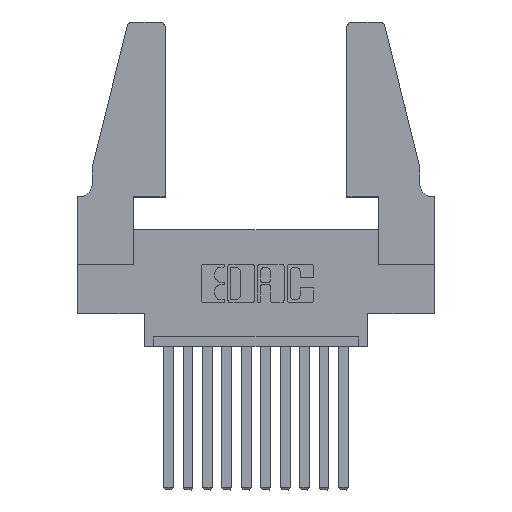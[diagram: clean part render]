
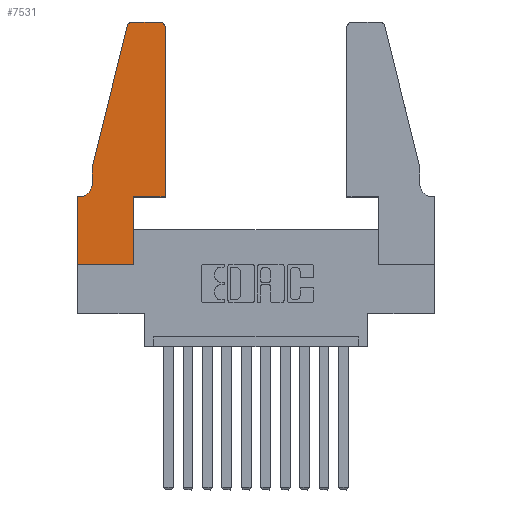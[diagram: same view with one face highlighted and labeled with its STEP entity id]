
A CAD part, top view. The second image highlights one B-rep face of the part: STEP entity #7531.
In plain terms, the highlighted planar face has unit normal (0, 0, 1).
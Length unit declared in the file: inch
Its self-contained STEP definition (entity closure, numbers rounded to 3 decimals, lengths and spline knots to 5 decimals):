
#400 = VERTEX_POINT ( 'NONE', #12386 ) ;
#505 = EDGE_CURVE ( 'NONE', #400, #11823, #3196, .T. ) ;
#638 = VERTEX_POINT ( 'NONE', #8035 ) ;
#693 = EDGE_CURVE ( 'NONE', #10097, #2169, #10620, .T. ) ;
#956 = DIRECTION ( 'NONE',  ( -1., 0., 0. ) ) ;
#965 = VERTEX_POINT ( 'NONE', #2497 ) ;
#1113 = CARTESIAN_POINT ( 'NONE',  ( 0.2605, 1.25, 0.37 ) ) ;
#1134 = CARTESIAN_POINT ( 'NONE',  ( 0.0755, 0.5, 0.37 ) ) ;
#1214 = CARTESIAN_POINT ( 'NONE',  ( 0.4205, 1.22, 0.37 ) ) ;
#1324 = LINE ( 'NONE', #4341, #2148 ) ;
#1554 = ORIENTED_EDGE ( 'NONE', *, *, #2371, .T. ) ;
#1599 = ORIENTED_EDGE ( 'NONE', *, *, #4383, .T. ) ;
#1638 = VECTOR ( 'NONE', #6532, 39.37008 ) ;
#1718 = ORIENTED_EDGE ( 'NONE', *, *, #505, .T. ) ;
#1797 = VECTOR ( 'NONE', #2634, 39.37008 ) ;
#1923 = CARTESIAN_POINT ( 'NONE',  ( 0., 0.35, 0.37 ) ) ;
#2148 = VECTOR ( 'NONE', #11804, 39.37008 ) ;
#2169 = VERTEX_POINT ( 'NONE', #2779 ) ;
#2243 = LINE ( 'NONE', #4639, #3432 ) ;
#2328 = LINE ( 'NONE', #1134, #8081 ) ;
#2371 = EDGE_CURVE ( 'NONE', #11823, #965, #11902, .T. ) ;
#2497 = CARTESIAN_POINT ( 'NONE',  ( 0.284, 1.25, 0.37 ) ) ;
#2634 = DIRECTION ( 'NONE',  ( -1., 0., 0. ) ) ;
#2743 = ORIENTED_EDGE ( 'NONE', *, *, #693, .T. ) ;
#2779 = CARTESIAN_POINT ( 'NONE',  ( 0.0055, 0.35, 0.37 ) ) ;
#2940 = EDGE_CURVE ( 'NONE', #2169, #9331, #7873, .T. ) ;
#3012 = ORIENTED_EDGE ( 'NONE', *, *, #10873, .T. ) ;
#3196 = CIRCLE ( 'NONE', #11890, 0.03 ) ;
#3250 = VECTOR ( 'NONE', #12392, 39.37008 ) ;
#3340 = CARTESIAN_POINT ( 'NONE',  ( 0.0755, 0.42, 0.37 ) ) ;
#3370 = ORIENTED_EDGE ( 'NONE', *, *, #13702, .T. ) ;
#3432 = VECTOR ( 'NONE', #3545, 39.37008 ) ;
#3545 = DIRECTION ( 'NONE',  ( 0., 1., 0. ) ) ;
#4165 = ORIENTED_EDGE ( 'NONE', *, *, #8785, .T. ) ;
#4227 = CARTESIAN_POINT ( 'NONE',  ( 0.25487, 1.22718, 0.37 ) ) ;
#4241 = DIRECTION ( 'NONE',  ( 0., 0., -1. ) ) ;
#4253 = ORIENTED_EDGE ( 'NONE', *, *, #2940, .T. ) ;
#4341 = CARTESIAN_POINT ( 'NONE',  ( 0., 0., 0.37 ) ) ;
#4377 = ORIENTED_EDGE ( 'NONE', *, *, #5348, .T. ) ;
#4383 = EDGE_CURVE ( 'NONE', #12755, #8589, #2243, .T. ) ;
#4432 = DIRECTION ( 'NONE',  ( 0., -1., 0. ) ) ;
#4639 = CARTESIAN_POINT ( 'NONE',  ( 0.2865, 0.35, 0.37 ) ) ;
#4692 = DIRECTION ( 'NONE',  ( 0., 0., 1. ) ) ;
#5131 = CARTESIAN_POINT ( 'NONE',  ( 0.4505, 0.35, 0.37 ) ) ;
#5348 = EDGE_CURVE ( 'NONE', #6345, #12755, #1324, .T. ) ;
#5394 = LINE ( 'NONE', #12073, #10742 ) ;
#5472 = CARTESIAN_POINT ( 'NONE',  ( 0.4205, 1.25, 0.37 ) ) ;
#5536 = CARTESIAN_POINT ( 'NONE',  ( 0.4505, 0.35, 0.37 ) ) ;
#5636 = LINE ( 'NONE', #5536, #9297 ) ;
#5782 = ORIENTED_EDGE ( 'NONE', *, *, #7987, .T. ) ;
#6209 = VERTEX_POINT ( 'NONE', #5131 ) ;
#6345 = VERTEX_POINT ( 'NONE', #7859 ) ;
#6377 = PLANE ( 'NONE',  #8987 ) ;
#6532 = DIRECTION ( 'NONE',  ( -1., 0., 0. ) ) ;
#6543 = CARTESIAN_POINT ( 'NONE',  ( 0.0755, 0.5, 0.37 ) ) ;
#6580 = AXIS2_PLACEMENT_3D ( 'NONE', #12140, #4692, #12188 ) ;
#6585 = DIRECTION ( 'NONE',  ( 1., 0., 0. ) ) ;
#6591 = DIRECTION ( 'NONE',  ( -0.239, -0.971, 0. ) ) ;
#6717 = AXIS2_PLACEMENT_3D ( 'NONE', #10223, #4241, #956 ) ;
#6825 = EDGE_CURVE ( 'NONE', #965, #8058, #13187, .T. ) ;
#7531 = ADVANCED_FACE ( 'NONE', ( #13856 ), #6377, .T. ) ;
#7621 = LINE ( 'NONE', #6543, #10789 ) ;
#7859 = CARTESIAN_POINT ( 'NONE',  ( 0., 0., 0.37 ) ) ;
#7873 = LINE ( 'NONE', #9066, #1797 ) ;
#7987 = EDGE_CURVE ( 'NONE', #6209, #400, #5636, .T. ) ;
#8035 = CARTESIAN_POINT ( 'NONE',  ( 0.0755, 0.5, 0.37 ) ) ;
#8058 = VERTEX_POINT ( 'NONE', #4227 ) ;
#8081 = VECTOR ( 'NONE', #6591, 39.37008 ) ;
#8177 = ORIENTED_EDGE ( 'NONE', *, *, #11136, .T. ) ;
#8589 = VERTEX_POINT ( 'NONE', #12774 ) ;
#8785 = EDGE_CURVE ( 'NONE', #638, #10097, #7621, .T. ) ;
#8933 = ORIENTED_EDGE ( 'NONE', *, *, #6825, .T. ) ;
#8987 = AXIS2_PLACEMENT_3D ( 'NONE', #12862, #9586, #9676 ) ;
#9066 = CARTESIAN_POINT ( 'NONE',  ( 0.0755, 0.35, 0.37 ) ) ;
#9234 = CARTESIAN_POINT ( 'NONE',  ( 0.2865, 0., 0.37 ) ) ;
#9297 = VECTOR ( 'NONE', #10866, 39.37008 ) ;
#9315 = LINE ( 'NONE', #13522, #3250 ) ;
#9331 = VERTEX_POINT ( 'NONE', #1923 ) ;
#9491 = EDGE_LOOP ( 'NONE', ( #1554, #8933, #3370, #4165, #2743, #4253, #3012, #4377, #1599, #8177, #5782, #1718 ) ) ;
#9586 = DIRECTION ( 'NONE',  ( 0., 0., 1. ) ) ;
#9676 = DIRECTION ( 'NONE',  ( 1., 0., 0. ) ) ;
#9712 = DIRECTION ( 'NONE',  ( 0., 0., 1. ) ) ;
#9856 = DIRECTION ( 'NONE',  ( 0., -1., 0. ) ) ;
#10097 = VERTEX_POINT ( 'NONE', #3340 ) ;
#10223 = CARTESIAN_POINT ( 'NONE',  ( 0.0055, 0.42, 0.37 ) ) ;
#10620 = CIRCLE ( 'NONE', #6717, 0.07 ) ;
#10742 = VECTOR ( 'NONE', #4432, 39.37008 ) ;
#10789 = VECTOR ( 'NONE', #9856, 39.37008 ) ;
#10866 = DIRECTION ( 'NONE',  ( 0., 1., 0. ) ) ;
#10873 = EDGE_CURVE ( 'NONE', #9331, #6345, #5394, .T. ) ;
#11136 = EDGE_CURVE ( 'NONE', #8589, #6209, #9315, .T. ) ;
#11804 = DIRECTION ( 'NONE',  ( 1., 0., 0. ) ) ;
#11823 = VERTEX_POINT ( 'NONE', #5472 ) ;
#11890 = AXIS2_PLACEMENT_3D ( 'NONE', #1214, #9712, #6585 ) ;
#11902 = LINE ( 'NONE', #1113, #1638 ) ;
#12073 = CARTESIAN_POINT ( 'NONE',  ( 0., 0., 0.37 ) ) ;
#12140 = CARTESIAN_POINT ( 'NONE',  ( 0.284, 1.22, 0.37 ) ) ;
#12188 = DIRECTION ( 'NONE',  ( 1., 0., 0. ) ) ;
#12386 = CARTESIAN_POINT ( 'NONE',  ( 0.4505, 1.22, 0.37 ) ) ;
#12392 = DIRECTION ( 'NONE',  ( 1., 0., 0. ) ) ;
#12755 = VERTEX_POINT ( 'NONE', #9234 ) ;
#12774 = CARTESIAN_POINT ( 'NONE',  ( 0.2865, 0.35, 0.37 ) ) ;
#12862 = CARTESIAN_POINT ( 'NONE',  ( 0., 0.35, 0.37 ) ) ;
#13187 = CIRCLE ( 'NONE', #6580, 0.03 ) ;
#13522 = CARTESIAN_POINT ( 'NONE',  ( 0.4505, 0.35, 0.37 ) ) ;
#13702 = EDGE_CURVE ( 'NONE', #8058, #638, #2328, .T. ) ;
#13856 = FACE_OUTER_BOUND ( 'NONE', #9491, .T. ) ;
